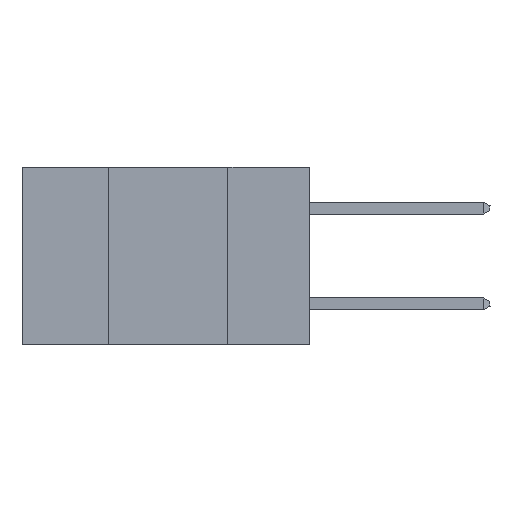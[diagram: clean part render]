
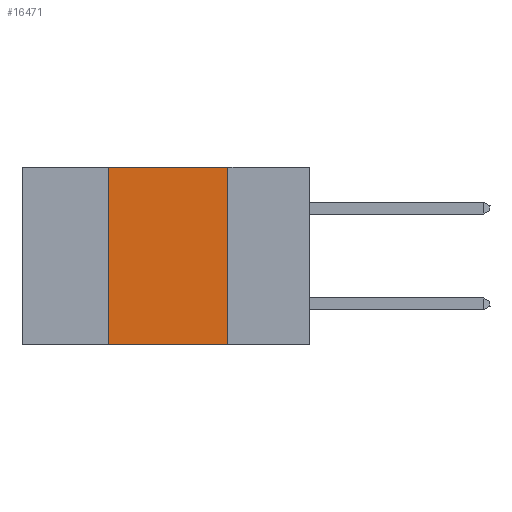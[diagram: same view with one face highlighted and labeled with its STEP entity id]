
A CAD part, left-side view. The second image highlights one B-rep face of the part: STEP entity #16471.
In plain terms, the highlighted planar face has unit normal (-1, 0, 0).
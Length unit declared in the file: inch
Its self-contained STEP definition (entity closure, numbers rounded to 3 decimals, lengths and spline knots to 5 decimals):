
#522 = LINE ( 'NONE', #1372, #20163 ) ;
#751 = VECTOR ( 'NONE', #19589, 39.37008 ) ;
#1372 = CARTESIAN_POINT ( 'NONE',  ( 0., 0.17, 0. ) ) ;
#2616 = FACE_OUTER_BOUND ( 'NONE', #13199, .T. ) ;
#3773 = LINE ( 'NONE', #21183, #16562 ) ;
#4125 = ORIENTED_EDGE ( 'NONE', *, *, #9118, .F. ) ;
#4653 = CARTESIAN_POINT ( 'NONE',  ( 0., 0.42, 0. ) ) ;
#5350 = CARTESIAN_POINT ( 'NONE',  ( 0., 0.17, -0.37 ) ) ;
#5511 = LINE ( 'NONE', #4653, #9951 ) ;
#5670 = PLANE ( 'NONE',  #17766 ) ;
#5784 = DIRECTION ( 'NONE',  ( 0., 0., -1. ) ) ;
#6573 = VERTEX_POINT ( 'NONE', #16776 ) ;
#7554 = CARTESIAN_POINT ( 'NONE',  ( 0., 0.42, 0. ) ) ;
#7832 = EDGE_CURVE ( 'NONE', #10130, #15430, #3773, .T. ) ;
#9118 = EDGE_CURVE ( 'NONE', #6573, #10130, #5511, .T. ) ;
#9933 = ORIENTED_EDGE ( 'NONE', *, *, #19003, .T. ) ;
#9951 = VECTOR ( 'NONE', #18046, 39.37008 ) ;
#10130 = VERTEX_POINT ( 'NONE', #7554 ) ;
#12499 = DIRECTION ( 'NONE',  ( 0., 0., -1. ) ) ;
#13199 = EDGE_LOOP ( 'NONE', ( #21503, #13588, #4125, #9933 ) ) ;
#13588 = ORIENTED_EDGE ( 'NONE', *, *, #7832, .F. ) ;
#13820 = LINE ( 'NONE', #23352, #751 ) ;
#15430 = VERTEX_POINT ( 'NONE', #24518 ) ;
#16471 = ADVANCED_FACE ( 'NONE', ( #2616 ), #5670, .F. ) ;
#16562 = VECTOR ( 'NONE', #22871, 39.37008 ) ;
#16776 = CARTESIAN_POINT ( 'NONE',  ( 0., 0.42, -0.37 ) ) ;
#17766 = AXIS2_PLACEMENT_3D ( 'NONE', #20027, #20776, #5784 ) ;
#18046 = DIRECTION ( 'NONE',  ( 0., 0., 1. ) ) ;
#19003 = EDGE_CURVE ( 'NONE', #6573, #24616, #13820, .T. ) ;
#19589 = DIRECTION ( 'NONE',  ( 0., -1., 0. ) ) ;
#20027 = CARTESIAN_POINT ( 'NONE',  ( 0., 0.6, 0. ) ) ;
#20163 = VECTOR ( 'NONE', #12499, 39.37008 ) ;
#20776 = DIRECTION ( 'NONE',  ( 1., 0., 0. ) ) ;
#21183 = CARTESIAN_POINT ( 'NONE',  ( 0., 0.6, 0. ) ) ;
#21503 = ORIENTED_EDGE ( 'NONE', *, *, #24505, .F. ) ;
#22871 = DIRECTION ( 'NONE',  ( 0., -1., 0. ) ) ;
#23352 = CARTESIAN_POINT ( 'NONE',  ( 0., 0.6, -0.37 ) ) ;
#24505 = EDGE_CURVE ( 'NONE', #15430, #24616, #522, .T. ) ;
#24518 = CARTESIAN_POINT ( 'NONE',  ( 0., 0.17, 0. ) ) ;
#24616 = VERTEX_POINT ( 'NONE', #5350 ) ;
